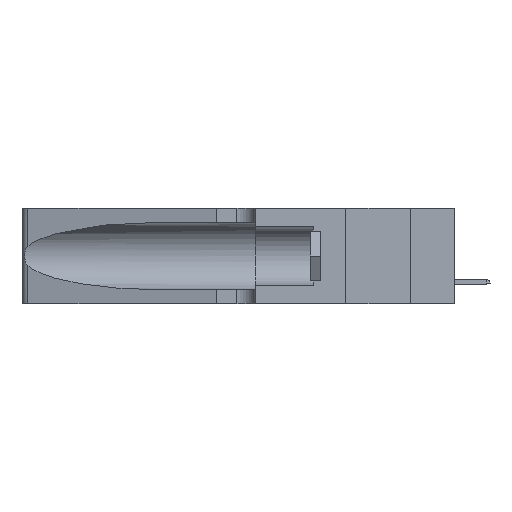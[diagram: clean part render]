
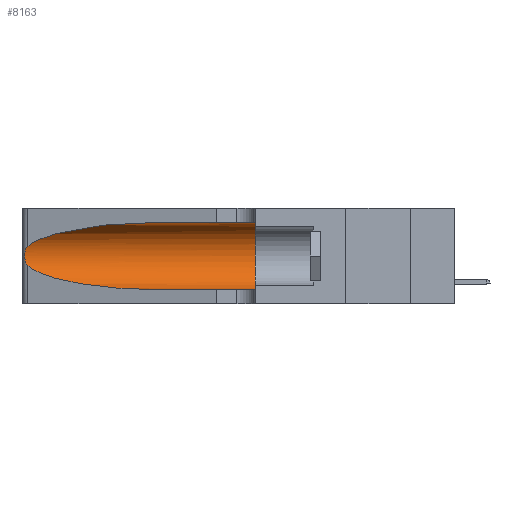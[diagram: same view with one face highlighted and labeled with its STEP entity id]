
A CAD part, left-side view. The second image highlights one B-rep face of the part: STEP entity #8163.
In plain terms, the highlighted cylindrical face has radius 3.308 mm (diameter 6.617 mm), a partial arc.
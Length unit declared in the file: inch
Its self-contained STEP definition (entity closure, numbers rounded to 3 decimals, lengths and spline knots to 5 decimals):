
#199 = FACE_OUTER_BOUND ( 'NONE', #3311, .T. ) ;
#259 = CARTESIAN_POINT ( 'NONE',  ( 0.25639, 1.23184, 0.21858 ) ) ;
#329 = VERTEX_POINT ( 'NONE', #10139 ) ;
#788 = EDGE_CURVE ( 'NONE', #2169, #11006, #16539, .T. ) ;
#1047 = LINE ( 'NONE', #5928, #3905 ) ;
#1311 = EDGE_CURVE ( 'NONE', #11006, #9588, #18487, .T. ) ;
#1379 = CARTESIAN_POINT ( 'NONE',  ( 0.18966, 0.96281, 0.05475 ) ) ;
#1598 = ORIENTED_EDGE ( 'NONE', *, *, #11625, .F. ) ;
#1648 = CARTESIAN_POINT ( 'NONE',  ( 0.25639, 1.23186, 0.15144 ) ) ;
#1957 = CARTESIAN_POINT ( 'NONE',  ( 0.26075, 1.23896, 0.178 ) ) ;
#2169 = VERTEX_POINT ( 'NONE', #4657 ) ;
#2960 = CARTESIAN_POINT ( 'NONE',  ( 0.2373, 1.15595, 0.08982 ) ) ;
#3311 = EDGE_LOOP ( 'NONE', ( #18886, #6627, #6541, #18421, #1598, #18477 ) ) ;
#3548 = CARTESIAN_POINT ( 'NONE',  ( 0.25854, 1.2359, 0.20912 ) ) ;
#3824 = EDGE_CURVE ( 'NONE', #12809, #329, #1047, .T. ) ;
#3905 = VECTOR ( 'NONE', #14144, 39.37008 ) ;
#4657 = CARTESIAN_POINT ( 'NONE',  ( 0.25487, 1.22718, 0.22369 ) ) ;
#5077 = CARTESIAN_POINT ( 'NONE',  ( 0.1305, 1.61858, 0.05475 ) ) ;
#5928 = CARTESIAN_POINT ( 'NONE',  ( 0.1305, 1.61858, 0.31525 ) ) ;
#6429 = CARTESIAN_POINT ( 'NONE',  ( 0.26017, 1.23833, 0.17102 ) ) ;
#6541 = ORIENTED_EDGE ( 'NONE', *, *, #1311, .T. ) ;
#6571 = CYLINDRICAL_SURFACE ( 'NONE', #14067, 0.13025 ) ;
#6578 = CARTESIAN_POINT ( 'NONE',  ( 0.2373, 1.15595, 0.28018 ) ) ;
#6623 = CARTESIAN_POINT ( 'NONE',  ( 0.25787, 1.23484, 0.2124 ) ) ;
#6627 = ORIENTED_EDGE ( 'NONE', *, *, #788, .T. ) ;
#6683 = CARTESIAN_POINT ( 'NONE',  ( 0.25487, 1.22718, 0.22369 ) ) ;
#6912 = CARTESIAN_POINT ( 'NONE',  ( 0.25487, 1.22718, 0.22369 ) ) ;
#7225 = CARTESIAN_POINT ( 'NONE',  ( 0.25487, 1.22718, 0.14631 ) ) ;
#7839 = CARTESIAN_POINT ( 'NONE',  ( 0.1305, 0.72297, 0.05475 ) ) ;
#8106 = CARTESIAN_POINT ( 'NONE',  ( 0.25555, 1.22993, 0.14849 ) ) ;
#8109 = CARTESIAN_POINT ( 'NONE',  ( 0.1305, 0.35, 0.185 ) ) ;
#8145 = DIRECTION ( 'NONE',  ( 0., -1., 0. ) ) ;
#8163 = ADVANCED_FACE ( 'NONE', ( #199 ), #6571, .F. ) ;
#8247 = VERTEX_POINT ( 'NONE', #17878 ) ;
#9457 = DIRECTION ( 'NONE',  ( 0., 0., -1. ) ) ;
#9473 = AXIS2_PLACEMENT_3D ( 'NONE', #8109, #16536, #9925 ) ;
#9588 = VERTEX_POINT ( 'NONE', #18105 ) ;
#9655 = LINE ( 'NONE', #5077, #20061 ) ;
#9925 = DIRECTION ( 'NONE',  ( 0., 0., 1. ) ) ;
#10023 = CARTESIAN_POINT ( 'NONE',  ( 0.25487, 1.22718, 0.14631 ) ) ;
#10139 = CARTESIAN_POINT ( 'NONE',  ( 0.1305, 0.35, 0.31525 ) ) ;
#10597 =( BOUNDED_CURVE ( )  B_SPLINE_CURVE ( 3, ( #11289, #17766, #6578, #6683 ),
 .UNSPECIFIED., .F., .F. ) 
 B_SPLINE_CURVE_WITH_KNOTS ( ( 4, 4 ),
 ( 1.5708, 2.84003 ),
 .UNSPECIFIED. ) 
 CURVE ( )  GEOMETRIC_REPRESENTATION_ITEM ( )  RATIONAL_B_SPLINE_CURVE ( ( 1., 0.87, 0.87, 1. ) ) 
 REPRESENTATION_ITEM ( '' )  );
#11006 = VERTEX_POINT ( 'NONE', #7225 ) ;
#11289 = CARTESIAN_POINT ( 'NONE',  ( 0.1305, 0.72297, 0.31525 ) ) ;
#11625 = EDGE_CURVE ( 'NONE', #329, #8247, #16622, .T. ) ;
#12809 = VERTEX_POINT ( 'NONE', #18812 ) ;
#12887 = DIRECTION ( 'NONE',  ( 0., -1., 0. ) ) ;
#13139 = CARTESIAN_POINT ( 'NONE',  ( 0.25856, 1.23593, 0.16098 ) ) ;
#13434 = CARTESIAN_POINT ( 'NONE',  ( 0.25555, 1.22994, 0.2215 ) ) ;
#14024 = EDGE_CURVE ( 'NONE', #9588, #8247, #9655, .T. ) ;
#14067 = AXIS2_PLACEMENT_3D ( 'NONE', #14689, #12887, #9457 ) ;
#14144 = DIRECTION ( 'NONE',  ( 0., -1., 0. ) ) ;
#14689 = CARTESIAN_POINT ( 'NONE',  ( 0.1305, 1.61858, 0.185 ) ) ;
#16233 = CARTESIAN_POINT ( 'NONE',  ( 0.26018, 1.23835, 0.19895 ) ) ;
#16536 = DIRECTION ( 'NONE',  ( 0., 1., 0. ) ) ;
#16539 = B_SPLINE_CURVE_WITH_KNOTS ( 'NONE', 3,
 ( #6912, #13434, #259, #6623, #3548, #16233, #19496, #1957, #6429, #13139, #19598, #1648, #8106, #10023 ),
 .UNSPECIFIED., .F., .F.,
 ( 4, 2, 2, 2, 2, 2, 4 ),
 ( 0., 0.00027, 0.00053, 0.00107, 0.0016, 0.00187, 0.00214 ),
 .UNSPECIFIED. ) ;
#16622 = CIRCLE ( 'NONE', #9473, 0.13025 ) ;
#17540 = CARTESIAN_POINT ( 'NONE',  ( 0.25487, 1.22718, 0.14631 ) ) ;
#17766 = CARTESIAN_POINT ( 'NONE',  ( 0.18966, 0.96281, 0.31525 ) ) ;
#17878 = CARTESIAN_POINT ( 'NONE',  ( 0.1305, 0.35, 0.05475 ) ) ;
#18105 = CARTESIAN_POINT ( 'NONE',  ( 0.1305, 0.72297, 0.05475 ) ) ;
#18421 = ORIENTED_EDGE ( 'NONE', *, *, #14024, .T. ) ;
#18477 = ORIENTED_EDGE ( 'NONE', *, *, #3824, .F. ) ;
#18487 =( BOUNDED_CURVE ( )  B_SPLINE_CURVE ( 3, ( #17540, #2960, #1379, #7839 ),
 .UNSPECIFIED., .F., .T. ) 
 B_SPLINE_CURVE_WITH_KNOTS ( ( 4, 4 ),
 ( 3.44316, 4.71239 ),
 .UNSPECIFIED. ) 
 CURVE ( )  GEOMETRIC_REPRESENTATION_ITEM ( )  RATIONAL_B_SPLINE_CURVE ( ( 1., 0.87, 0.87, 1. ) ) 
 REPRESENTATION_ITEM ( '' )  );
#18812 = CARTESIAN_POINT ( 'NONE',  ( 0.1305, 0.72297, 0.31525 ) ) ;
#18886 = ORIENTED_EDGE ( 'NONE', *, *, #19083, .T. ) ;
#19083 = EDGE_CURVE ( 'NONE', #12809, #2169, #10597, .T. ) ;
#19496 = CARTESIAN_POINT ( 'NONE',  ( 0.26075, 1.23896, 0.19203 ) ) ;
#19598 = CARTESIAN_POINT ( 'NONE',  ( 0.25789, 1.23486, 0.15765 ) ) ;
#20061 = VECTOR ( 'NONE', #8145, 39.37008 ) ;
